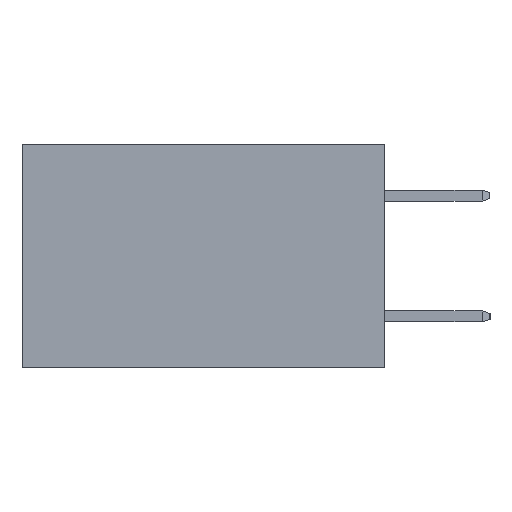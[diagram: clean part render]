
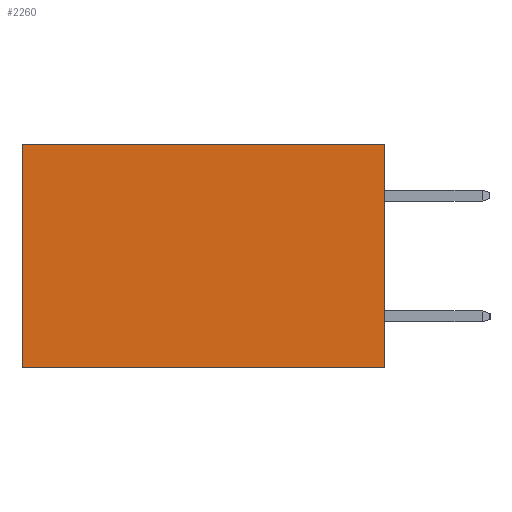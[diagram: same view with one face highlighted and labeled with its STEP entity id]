
A CAD part, left-side view. The second image highlights one B-rep face of the part: STEP entity #2260.
In plain terms, the highlighted planar face has unit normal (-1, 0, 0).
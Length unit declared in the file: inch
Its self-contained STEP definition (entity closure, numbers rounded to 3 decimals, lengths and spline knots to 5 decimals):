
#1555 = VECTOR ( 'NONE', #7176, 39.37008 ) ;
#1797 = CARTESIAN_POINT ( 'NONE',  ( 0.2615, 0., -0.37 ) ) ;
#1986 = DIRECTION ( 'NONE',  ( 0., 0., -1. ) ) ;
#2208 = VERTEX_POINT ( 'NONE', #2670 ) ;
#2226 = CARTESIAN_POINT ( 'NONE',  ( 0.2615, 0.6, -0.37 ) ) ;
#2260 = ADVANCED_FACE ( 'NONE', ( #10677 ), #11168, .F. ) ;
#2407 = DIRECTION ( 'NONE',  ( 0., 1., 0. ) ) ;
#2434 = CARTESIAN_POINT ( 'NONE',  ( 0.2615, 0., -0.37 ) ) ;
#2638 = ORIENTED_EDGE ( 'NONE', *, *, #3103, .F. ) ;
#2670 = CARTESIAN_POINT ( 'NONE',  ( 0.2615, 0.6, -0.37 ) ) ;
#2720 = ORIENTED_EDGE ( 'NONE', *, *, #10341, .T. ) ;
#3103 = EDGE_CURVE ( 'NONE', #5274, #2208, #4147, .T. ) ;
#3337 = EDGE_CURVE ( 'NONE', #10468, #5274, #10412, .T. ) ;
#4050 = LINE ( 'NONE', #2226, #6374 ) ;
#4147 = LINE ( 'NONE', #2434, #8366 ) ;
#4609 = CARTESIAN_POINT ( 'NONE',  ( 0.2615, 0., 0. ) ) ;
#5274 = VERTEX_POINT ( 'NONE', #7560 ) ;
#5784 = VECTOR ( 'NONE', #1986, 39.37008 ) ;
#6352 = LINE ( 'NONE', #4609, #1555 ) ;
#6374 = VECTOR ( 'NONE', #8189, 39.37008 ) ;
#6443 = ORIENTED_EDGE ( 'NONE', *, *, #3337, .F. ) ;
#7125 = CARTESIAN_POINT ( 'NONE',  ( 0.2615, 0.6, 0. ) ) ;
#7176 = DIRECTION ( 'NONE',  ( 0., 1., 0. ) ) ;
#7311 = CARTESIAN_POINT ( 'NONE',  ( 0.2615, 0., 0. ) ) ;
#7560 = CARTESIAN_POINT ( 'NONE',  ( 0.2615, 0., -0.37 ) ) ;
#8189 = DIRECTION ( 'NONE',  ( 0., 0., -1. ) ) ;
#8366 = VECTOR ( 'NONE', #2407, 39.37008 ) ;
#8646 = AXIS2_PLACEMENT_3D ( 'NONE', #11282, #11141, #11104 ) ;
#8805 = VERTEX_POINT ( 'NONE', #7125 ) ;
#9086 = EDGE_CURVE ( 'NONE', #8805, #2208, #4050, .T. ) ;
#9892 = ORIENTED_EDGE ( 'NONE', *, *, #9086, .T. ) ;
#10341 = EDGE_CURVE ( 'NONE', #10468, #8805, #6352, .T. ) ;
#10412 = LINE ( 'NONE', #1797, #5784 ) ;
#10468 = VERTEX_POINT ( 'NONE', #7311 ) ;
#10610 = EDGE_LOOP ( 'NONE', ( #9892, #2638, #6443, #2720 ) ) ;
#10677 = FACE_OUTER_BOUND ( 'NONE', #10610, .T. ) ;
#11104 = DIRECTION ( 'NONE',  ( 0., 0., -1. ) ) ;
#11141 = DIRECTION ( 'NONE',  ( 1., 0., 0. ) ) ;
#11168 = PLANE ( 'NONE',  #8646 ) ;
#11282 = CARTESIAN_POINT ( 'NONE',  ( 0.2615, 0., -0.37 ) ) ;
